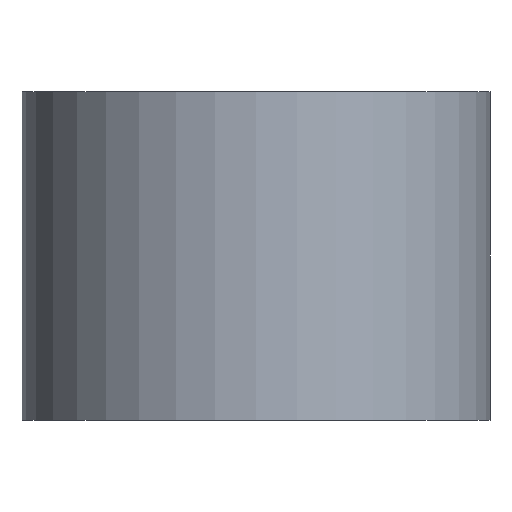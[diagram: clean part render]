
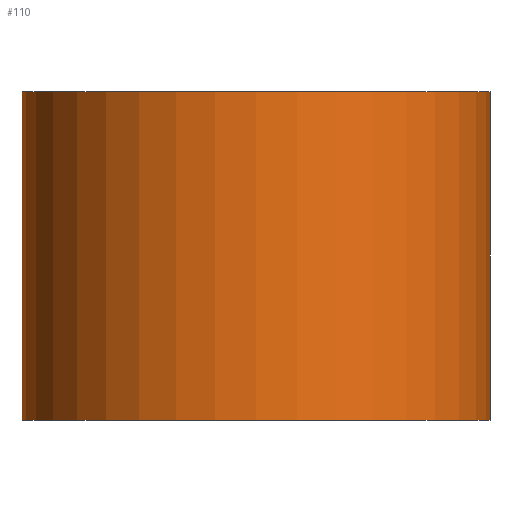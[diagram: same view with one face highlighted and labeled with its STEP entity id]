
A CAD part, front view. The second image highlights one B-rep face of the part: STEP entity #110.
In plain terms, the highlighted cylindrical face has radius 5.715 mm (diameter 11.43 mm), a partial arc.
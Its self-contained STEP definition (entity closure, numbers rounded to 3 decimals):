
#2 = ORIENTED_EDGE ( 'NONE', *, *, #198, .F. ) ;
#5 = AXIS2_PLACEMENT_3D ( 'NONE', #207, #206, #200 ) ;
#8 = VERTEX_POINT ( 'NONE', #18 ) ;
#11 = DIRECTION ( 'NONE',  ( 0., 0., -1. ) ) ;
#12 = LINE ( 'NONE', #14, #117 ) ;
#14 = CARTESIAN_POINT ( 'NONE',  ( 5.715, 0., 16.164 ) ) ;
#18 = CARTESIAN_POINT ( 'NONE',  ( -5.715, 0., 0. ) ) ;
#22 = AXIS2_PLACEMENT_3D ( 'NONE', #210, #11, #209 ) ;
#29 = LINE ( 'NONE', #179, #68 ) ;
#32 = CYLINDRICAL_SURFACE ( 'NONE', #22, 5.715 ) ;
#35 = AXIS2_PLACEMENT_3D ( 'NONE', #132, #130, #129 ) ;
#38 = CARTESIAN_POINT ( 'NONE',  ( 5.715, 0., 0. ) ) ;
#44 = CIRCLE ( 'NONE', #35, 5.715 ) ;
#62 = VERTEX_POINT ( 'NONE', #142 ) ;
#63 = VERTEX_POINT ( 'NONE', #38 ) ;
#68 = VECTOR ( 'NONE', #175, 1000. ) ;
#70 = CIRCLE ( 'NONE', #5, 5.715 ) ;
#71 = EDGE_LOOP ( 'NONE', ( #193, #184, #94, #2 ) ) ;
#84 = VERTEX_POINT ( 'NONE', #178 ) ;
#94 = ORIENTED_EDGE ( 'NONE', *, *, #118, .T. ) ;
#97 = EDGE_CURVE ( 'NONE', #63, #84, #12, .T. ) ;
#108 = EDGE_CURVE ( 'NONE', #8, #63, #70, .T. ) ;
#110 = ADVANCED_FACE ( 'NONE', ( #165 ), #32, .T. ) ;
#117 = VECTOR ( 'NONE', #214, 1000. ) ;
#118 = EDGE_CURVE ( 'NONE', #8, #62, #29, .T. ) ;
#129 = DIRECTION ( 'NONE',  ( -1., 0., 0. ) ) ;
#130 = DIRECTION ( 'NONE',  ( 0., 0., -1. ) ) ;
#132 = CARTESIAN_POINT ( 'NONE',  ( 0., 0., -8.026 ) ) ;
#142 = CARTESIAN_POINT ( 'NONE',  ( -5.715, 0., -8.026 ) ) ;
#165 = FACE_OUTER_BOUND ( 'NONE', #71, .T. ) ;
#175 = DIRECTION ( 'NONE',  ( 0., 0., -1. ) ) ;
#178 = CARTESIAN_POINT ( 'NONE',  ( 5.715, 0., -8.026 ) ) ;
#179 = CARTESIAN_POINT ( 'NONE',  ( -5.715, 0., 16.164 ) ) ;
#184 = ORIENTED_EDGE ( 'NONE', *, *, #108, .F. ) ;
#193 = ORIENTED_EDGE ( 'NONE', *, *, #97, .F. ) ;
#198 = EDGE_CURVE ( 'NONE', #84, #62, #44, .T. ) ;
#200 = DIRECTION ( 'NONE',  ( -1., 0., 0. ) ) ;
#206 = DIRECTION ( 'NONE',  ( 0., 0., 1. ) ) ;
#207 = CARTESIAN_POINT ( 'NONE',  ( 0., 0., 0. ) ) ;
#209 = DIRECTION ( 'NONE',  ( -1., 0., 0. ) ) ;
#210 = CARTESIAN_POINT ( 'NONE',  ( 0., 0., 16.164 ) ) ;
#214 = DIRECTION ( 'NONE',  ( 0., 0., -1. ) ) ;
